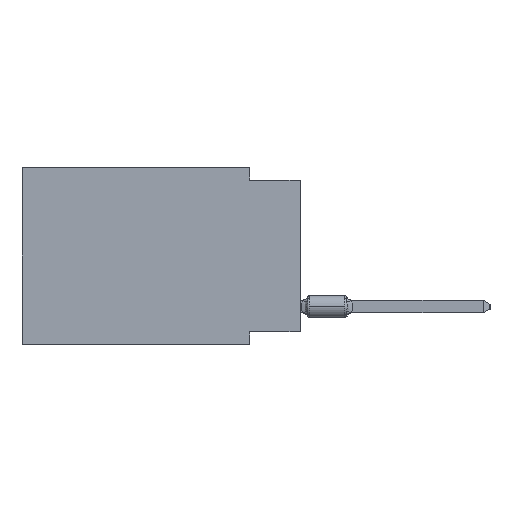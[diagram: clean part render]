
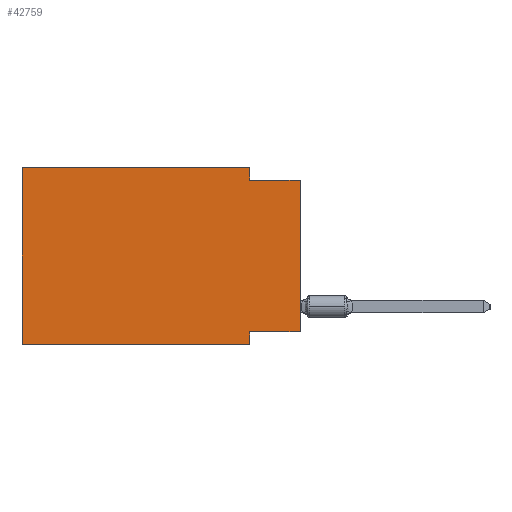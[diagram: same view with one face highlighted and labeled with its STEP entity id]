
A CAD part, left-side view. The second image highlights one B-rep face of the part: STEP entity #42759.
In plain terms, the highlighted planar face has unit normal (-1, 0, 0).
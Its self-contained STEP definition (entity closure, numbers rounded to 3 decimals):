
#113 = LINE ( 'NONE', #40820, #76174 ) ;
#1727 = CARTESIAN_POINT ( 'NONE',  ( 0., 13.97, 0. ) ) ;
#9648 = CARTESIAN_POINT ( 'NONE',  ( 0., 13.97, -8.89 ) ) ;
#10754 = DIRECTION ( 'NONE',  ( 0., -1., 0. ) ) ;
#13651 = VECTOR ( 'NONE', #10754, 1000. ) ;
#17207 = CARTESIAN_POINT ( 'NONE',  ( 0., 2.54, 0. ) ) ;
#17583 = VECTOR ( 'NONE', #29121, 1000. ) ;
#21463 = VERTEX_POINT ( 'NONE', #108354 ) ;
#23946 = CARTESIAN_POINT ( 'NONE',  ( 0., 2.54, -8.89 ) ) ;
#25103 = VECTOR ( 'NONE', #101439, 1000. ) ;
#26819 = EDGE_CURVE ( 'NONE', #95919, #39499, #43559, .T. ) ;
#29121 = DIRECTION ( 'NONE',  ( 0., 0., 1. ) ) ;
#29842 = CARTESIAN_POINT ( 'NONE',  ( 0., 0., -8.255 ) ) ;
#31870 = DIRECTION ( 'NONE',  ( 0., 0., -1. ) ) ;
#33642 = DIRECTION ( 'NONE',  ( 0., 1., 0. ) ) ;
#34345 = ORIENTED_EDGE ( 'NONE', *, *, #107390, .F. ) ;
#34498 = LINE ( 'NONE', #9648, #13651 ) ;
#35354 = VERTEX_POINT ( 'NONE', #63007 ) ;
#39499 = VERTEX_POINT ( 'NONE', #86625 ) ;
#40820 = CARTESIAN_POINT ( 'NONE',  ( 0., 13.97, 0. ) ) ;
#42759 = ADVANCED_FACE ( 'NONE', ( #97133 ), #63217, .F. ) ;
#43559 = LINE ( 'NONE', #111398, #68021 ) ;
#48212 = ORIENTED_EDGE ( 'NONE', *, *, #26819, .F. ) ;
#52995 = EDGE_CURVE ( 'NONE', #35354, #60173, #59349, .T. ) ;
#53796 = VECTOR ( 'NONE', #75756, 1000. ) ;
#55356 = VERTEX_POINT ( 'NONE', #98229 ) ;
#57684 = AXIS2_PLACEMENT_3D ( 'NONE', #107299, #71709, #80726 ) ;
#58305 = DIRECTION ( 'NONE',  ( 0., -1., 0. ) ) ;
#59349 = LINE ( 'NONE', #59899, #53796 ) ;
#59899 = CARTESIAN_POINT ( 'NONE',  ( 0., 13.97, 0. ) ) ;
#60173 = VERTEX_POINT ( 'NONE', #1727 ) ;
#61682 = ORIENTED_EDGE ( 'NONE', *, *, #79066, .F. ) ;
#63007 = CARTESIAN_POINT ( 'NONE',  ( 0., 13.97, -8.89 ) ) ;
#63217 = PLANE ( 'NONE',  #57684 ) ;
#63554 = CARTESIAN_POINT ( 'NONE',  ( 0., 0., 0. ) ) ;
#68021 = VECTOR ( 'NONE', #77461, 1000. ) ;
#69030 = EDGE_CURVE ( 'NONE', #69976, #55356, #107086, .T. ) ;
#69976 = VERTEX_POINT ( 'NONE', #29842 ) ;
#71684 = EDGE_CURVE ( 'NONE', #39499, #55356, #86143, .T. ) ;
#71709 = DIRECTION ( 'NONE',  ( 1., 0., 0. ) ) ;
#74318 = CARTESIAN_POINT ( 'NONE',  ( 0., 0., -8.255 ) ) ;
#75756 = DIRECTION ( 'NONE',  ( 0., 0., 1. ) ) ;
#75903 = LINE ( 'NONE', #23946, #100170 ) ;
#76003 = CARTESIAN_POINT ( 'NONE',  ( 0., 0., -0.635 ) ) ;
#76174 = VECTOR ( 'NONE', #58305, 1000. ) ;
#77461 = DIRECTION ( 'NONE',  ( 0., 0., -1. ) ) ;
#79066 = EDGE_CURVE ( 'NONE', #69976, #21463, #84455, .T. ) ;
#80726 = DIRECTION ( 'NONE',  ( 0., 0., -1. ) ) ;
#83412 = ORIENTED_EDGE ( 'NONE', *, *, #103690, .T. ) ;
#84455 = LINE ( 'NONE', #74318, #85550 ) ;
#85550 = VECTOR ( 'NONE', #33642, 1000. ) ;
#86143 = LINE ( 'NONE', #76003, #25103 ) ;
#86625 = CARTESIAN_POINT ( 'NONE',  ( 0., 2.54, -0.635 ) ) ;
#92426 = ORIENTED_EDGE ( 'NONE', *, *, #103145, .F. ) ;
#95919 = VERTEX_POINT ( 'NONE', #17207 ) ;
#97133 = FACE_OUTER_BOUND ( 'NONE', #107836, .T. ) ;
#98229 = CARTESIAN_POINT ( 'NONE',  ( 0., 0., -0.635 ) ) ;
#98364 = ORIENTED_EDGE ( 'NONE', *, *, #71684, .F. ) ;
#100170 = VECTOR ( 'NONE', #31870, 1000. ) ;
#101439 = DIRECTION ( 'NONE',  ( 0., -1., 0. ) ) ;
#103145 = EDGE_CURVE ( 'NONE', #21463, #105952, #75903, .T. ) ;
#103690 = EDGE_CURVE ( 'NONE', #35354, #105952, #34498, .T. ) ;
#105952 = VERTEX_POINT ( 'NONE', #108052 ) ;
#107086 = LINE ( 'NONE', #63554, #17583 ) ;
#107140 = ORIENTED_EDGE ( 'NONE', *, *, #52995, .F. ) ;
#107299 = CARTESIAN_POINT ( 'NONE',  ( 0., 13.97, 0. ) ) ;
#107390 = EDGE_CURVE ( 'NONE', #60173, #95919, #113, .T. ) ;
#107836 = EDGE_LOOP ( 'NONE', ( #109731, #98364, #48212, #34345, #107140, #83412, #92426, #61682 ) ) ;
#108052 = CARTESIAN_POINT ( 'NONE',  ( 0., 2.54, -8.89 ) ) ;
#108354 = CARTESIAN_POINT ( 'NONE',  ( 0., 2.54, -8.255 ) ) ;
#109731 = ORIENTED_EDGE ( 'NONE', *, *, #69030, .T. ) ;
#111398 = CARTESIAN_POINT ( 'NONE',  ( 0., 2.54, 0. ) ) ;
